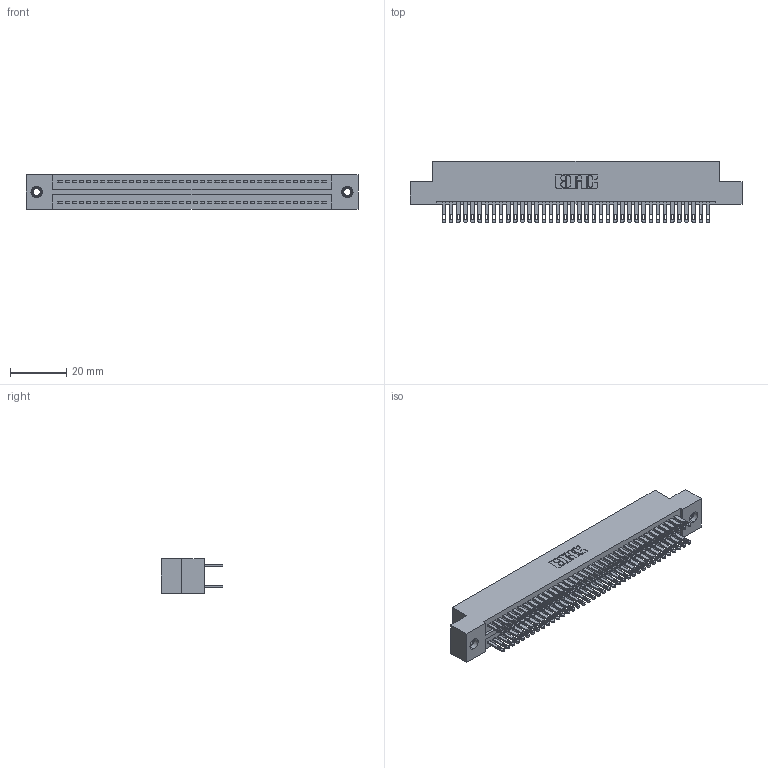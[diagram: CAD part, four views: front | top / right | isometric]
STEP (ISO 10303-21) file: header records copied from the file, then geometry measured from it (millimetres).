
FILE_DESCRIPTION (( 'STEP AP203' ), '1' );
FILE_NAME ('325-076-500-207.STEP', '2020-02-25T04:12:33', ( '' ), ( '' ), 'SwSTEP 2.0', 'SolidWorks 2016', '' );
FILE_SCHEMA (( 'CONFIG_CONTROL_DESIGN' ));
Length unit declared in the file: inch
Products named in the file (4): 345-250-001_345-250-005-103; 325-292-001_325-293-100; 325 Part_TI; 325-076-500-207
Assembly tree (79 placements, depth 2):
  325-076-500-207
    325 Part_TI
    325-292-001_325-293-100  x76
    345-250-001_345-250-005-103  x2
Bounding box: 118.24 x 21.84 x 12.45 mm (x, y, z)
Volume: 15446.7 mm3; surface area: 19422.3 mm2
Topology: 79 solids, 79 shells, 3822 faces, 11619 edges, 7738 vertices
Faces by surface type: plane 2382, cylinder 1424, cone 12, torus 4
Entity records: 26080 total; most frequent: CARTESIAN_POINT 4309, ORIENTED_EDGE 4238, DIRECTION 3721, EDGE_CURVE 2119, VECTOR 1967, LINE 1967, VERTEX_POINT 1408, AXIS2_PLACEMENT_3D 877
